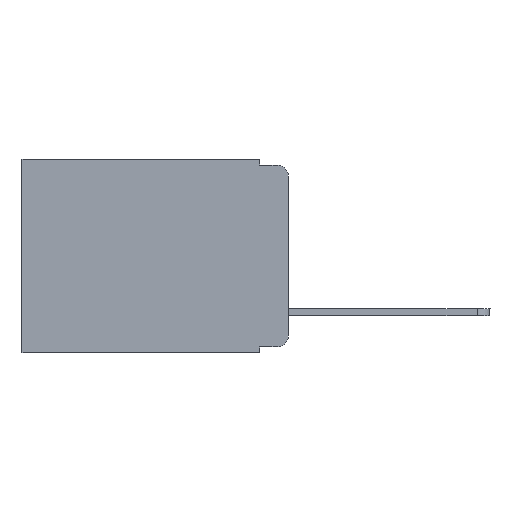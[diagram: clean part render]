
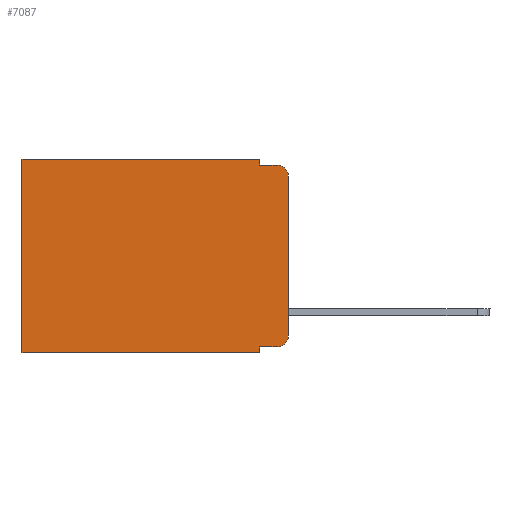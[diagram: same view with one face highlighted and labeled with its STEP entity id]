
A CAD part, left-side view. The second image highlights one B-rep face of the part: STEP entity #7087.
In plain terms, the highlighted planar face has unit normal (-1, 0, 0).
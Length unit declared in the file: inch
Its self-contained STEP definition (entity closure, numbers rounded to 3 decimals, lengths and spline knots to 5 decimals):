
#18 = DIRECTION ( 'NONE',  ( -1., 0., 0. ) ) ;
#603 = LINE ( 'NONE', #2452, #10651 ) ;
#724 = CARTESIAN_POINT ( 'NONE',  ( 0.298, 0.02, -0.01 ) ) ;
#908 = DIRECTION ( 'NONE',  ( 0., 0., -1. ) ) ;
#1192 = AXIS2_PLACEMENT_3D ( 'NONE', #5683, #12219, #908 ) ;
#1361 = EDGE_CURVE ( 'NONE', #4065, #6997, #5988, .T. ) ;
#1518 = CARTESIAN_POINT ( 'NONE',  ( 0.298, 0., 0. ) ) ;
#1761 = VERTEX_POINT ( 'NONE', #724 ) ;
#1783 = DIRECTION ( 'NONE',  ( 0., 0., -1. ) ) ;
#1835 = PLANE ( 'NONE',  #1192 ) ;
#1975 = VECTOR ( 'NONE', #9848, 39.37008 ) ;
#1998 = CARTESIAN_POINT ( 'NONE',  ( 0.298, 0.051, 0. ) ) ;
#2019 = FACE_OUTER_BOUND ( 'NONE', #9095, .T. ) ;
#2290 = DIRECTION ( 'NONE',  ( 0., 0., -1. ) ) ;
#2381 = LINE ( 'NONE', #1518, #5406 ) ;
#2452 = CARTESIAN_POINT ( 'NONE',  ( 0.298, 0., 0. ) ) ;
#2502 = DIRECTION ( 'NONE',  ( 0., 0., -1. ) ) ;
#2566 = VERTEX_POINT ( 'NONE', #8330 ) ;
#2642 = EDGE_CURVE ( 'NONE', #8354, #1761, #10307, .T. ) ;
#2721 = ORIENTED_EDGE ( 'NONE', *, *, #1361, .T. ) ;
#2866 = CARTESIAN_POINT ( 'NONE',  ( 0.298, 0.051, -0.333 ) ) ;
#2876 = LINE ( 'NONE', #1998, #9178 ) ;
#2910 = CARTESIAN_POINT ( 'NONE',  ( 0.298, 0.051, 0. ) ) ;
#3049 = CARTESIAN_POINT ( 'NONE',  ( 0.298, 0.473, 0. ) ) ;
#3227 = EDGE_CURVE ( 'NONE', #7252, #8029, #10780, .T. ) ;
#3763 = VECTOR ( 'NONE', #11386, 39.37008 ) ;
#3802 = DIRECTION ( 'NONE',  ( 0., 0., -1. ) ) ;
#3966 = EDGE_CURVE ( 'NONE', #2566, #1761, #9287, .T. ) ;
#4065 = VERTEX_POINT ( 'NONE', #4972 ) ;
#4237 = AXIS2_PLACEMENT_3D ( 'NONE', #10931, #11860, #1783 ) ;
#4725 = VERTEX_POINT ( 'NONE', #5498 ) ;
#4972 = CARTESIAN_POINT ( 'NONE',  ( 0.298, 0.02, -0.333 ) ) ;
#5385 = VECTOR ( 'NONE', #6567, 39.37008 ) ;
#5406 = VECTOR ( 'NONE', #8251, 39.37008 ) ;
#5496 = ORIENTED_EDGE ( 'NONE', *, *, #2642, .F. ) ;
#5498 = CARTESIAN_POINT ( 'NONE',  ( 0.298, 0.473, 0. ) ) ;
#5549 = CARTESIAN_POINT ( 'NONE',  ( 0.298, 0.051, -0.333 ) ) ;
#5630 = ORIENTED_EDGE ( 'NONE', *, *, #5729, .T. ) ;
#5683 = CARTESIAN_POINT ( 'NONE',  ( 0.298, 0., 0. ) ) ;
#5729 = EDGE_CURVE ( 'NONE', #8481, #4725, #603, .T. ) ;
#5988 = CIRCLE ( 'NONE', #4237, 0.02 ) ;
#6031 = CARTESIAN_POINT ( 'NONE',  ( 0.298, 0., -0.343 ) ) ;
#6231 = DIRECTION ( 'NONE',  ( 0., 1., 0. ) ) ;
#6564 = ORIENTED_EDGE ( 'NONE', *, *, #3966, .T. ) ;
#6567 = DIRECTION ( 'NONE',  ( 0., -1., 0. ) ) ;
#6997 = VERTEX_POINT ( 'NONE', #11047 ) ;
#7087 = ADVANCED_FACE ( 'NONE', ( #2019 ), #1835, .F. ) ;
#7133 = LINE ( 'NONE', #8359, #7601 ) ;
#7168 = CARTESIAN_POINT ( 'NONE',  ( 0.298, 0.051, -0.01 ) ) ;
#7252 = VERTEX_POINT ( 'NONE', #9669 ) ;
#7496 = VERTEX_POINT ( 'NONE', #5549 ) ;
#7601 = VECTOR ( 'NONE', #2502, 39.37008 ) ;
#7851 = ORIENTED_EDGE ( 'NONE', *, *, #11943, .F. ) ;
#7999 = EDGE_CURVE ( 'NONE', #7496, #4065, #10447, .T. ) ;
#8029 = VERTEX_POINT ( 'NONE', #10211 ) ;
#8251 = DIRECTION ( 'NONE',  ( 0., 0., -1. ) ) ;
#8330 = CARTESIAN_POINT ( 'NONE',  ( 0.298, 0., -0.03 ) ) ;
#8349 = ORIENTED_EDGE ( 'NONE', *, *, #9019, .F. ) ;
#8354 = VERTEX_POINT ( 'NONE', #7168 ) ;
#8359 = CARTESIAN_POINT ( 'NONE',  ( 0.298, 0.051, 0. ) ) ;
#8448 = CARTESIAN_POINT ( 'NONE',  ( 0.298, 0.051, -0.01 ) ) ;
#8462 = CARTESIAN_POINT ( 'NONE',  ( 0.298, 0.02, -0.03 ) ) ;
#8481 = VERTEX_POINT ( 'NONE', #2910 ) ;
#9019 = EDGE_CURVE ( 'NONE', #2566, #6997, #2381, .T. ) ;
#9095 = EDGE_LOOP ( 'NONE', ( #8349, #6564, #5496, #10522, #5630, #9534, #11814, #7851, #11243, #2721 ) ) ;
#9178 = VECTOR ( 'NONE', #9527, 39.37008 ) ;
#9287 = CIRCLE ( 'NONE', #9479, 0.02 ) ;
#9479 = AXIS2_PLACEMENT_3D ( 'NONE', #8462, #18, #3802 ) ;
#9527 = DIRECTION ( 'NONE',  ( 0., 0., -1. ) ) ;
#9534 = ORIENTED_EDGE ( 'NONE', *, *, #9739, .T. ) ;
#9669 = CARTESIAN_POINT ( 'NONE',  ( 0.298, 0.051, -0.343 ) ) ;
#9739 = EDGE_CURVE ( 'NONE', #4725, #8029, #10755, .T. ) ;
#9848 = DIRECTION ( 'NONE',  ( 0., 1., 0. ) ) ;
#10211 = CARTESIAN_POINT ( 'NONE',  ( 0.298, 0.473, -0.343 ) ) ;
#10307 = LINE ( 'NONE', #8448, #3763 ) ;
#10447 = LINE ( 'NONE', #2866, #5385 ) ;
#10522 = ORIENTED_EDGE ( 'NONE', *, *, #12157, .F. ) ;
#10651 = VECTOR ( 'NONE', #6231, 39.37008 ) ;
#10755 = LINE ( 'NONE', #3049, #11320 ) ;
#10780 = LINE ( 'NONE', #6031, #1975 ) ;
#10931 = CARTESIAN_POINT ( 'NONE',  ( 0.298, 0.02, -0.313 ) ) ;
#11047 = CARTESIAN_POINT ( 'NONE',  ( 0.298, 0., -0.313 ) ) ;
#11243 = ORIENTED_EDGE ( 'NONE', *, *, #7999, .T. ) ;
#11320 = VECTOR ( 'NONE', #2290, 39.37008 ) ;
#11386 = DIRECTION ( 'NONE',  ( 0., -1., 0. ) ) ;
#11814 = ORIENTED_EDGE ( 'NONE', *, *, #3227, .F. ) ;
#11860 = DIRECTION ( 'NONE',  ( -1., 0., 0. ) ) ;
#11943 = EDGE_CURVE ( 'NONE', #7496, #7252, #7133, .T. ) ;
#12157 = EDGE_CURVE ( 'NONE', #8481, #8354, #2876, .T. ) ;
#12219 = DIRECTION ( 'NONE',  ( 1., 0., 0. ) ) ;
